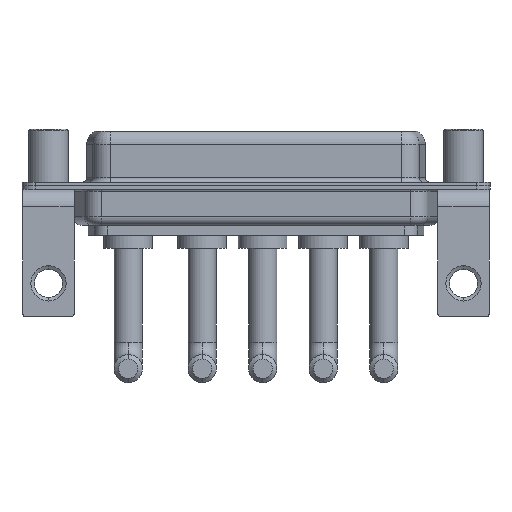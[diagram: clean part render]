
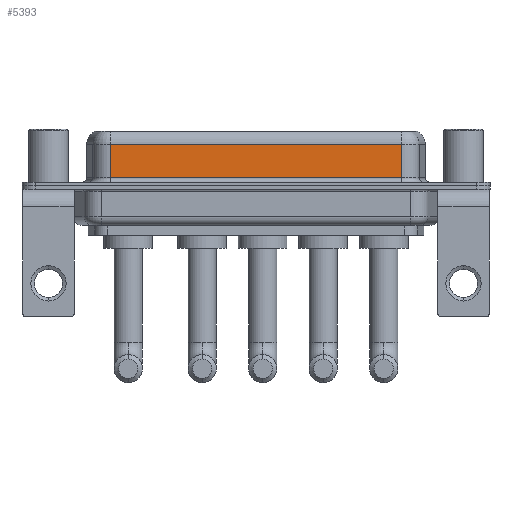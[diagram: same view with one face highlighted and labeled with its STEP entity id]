
A CAD part, front view. The second image highlights one B-rep face of the part: STEP entity #5393.
In plain terms, the highlighted planar face has unit normal (0, -1, 0).
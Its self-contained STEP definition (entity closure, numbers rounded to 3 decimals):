
#1314 = VECTOR ( 'NONE', #11670, 1000. ) ;
#1355 = CARTESIAN_POINT ( 'NONE',  ( 40.037, -3.95, 0.9 ) ) ;
#1744 = PLANE ( 'NONE',  #7026 ) ;
#2052 = CARTESIAN_POINT ( 'NONE',  ( 7.013, -3.95, 0.9 ) ) ;
#2108 = EDGE_CURVE ( 'NONE', #8559, #7716, #10728, .T. ) ;
#2201 = ORIENTED_EDGE ( 'NONE', *, *, #2108, .T. ) ;
#2359 = CARTESIAN_POINT ( 'NONE',  ( 40.037, -3.95, 4.65 ) ) ;
#2680 = VECTOR ( 'NONE', #7348, 1000. ) ;
#4213 = LINE ( 'NONE', #5383, #14626 ) ;
#4260 = EDGE_CURVE ( 'NONE', #7000, #5356, #11518, .T. ) ;
#4943 = EDGE_CURVE ( 'NONE', #8559, #5356, #4213, .T. ) ;
#5019 = CARTESIAN_POINT ( 'NONE',  ( 40.037, -3.95, 4.65 ) ) ;
#5356 = VERTEX_POINT ( 'NONE', #1355 ) ;
#5383 = CARTESIAN_POINT ( 'NONE',  ( 40.037, -3.95, 6.4 ) ) ;
#5393 = ADVANCED_FACE ( 'NONE', ( #11448 ), #1744, .F. ) ;
#5395 = EDGE_LOOP ( 'NONE', ( #12121, #2201, #13074, #6620 ) ) ;
#5891 = VECTOR ( 'NONE', #14658, 1000. ) ;
#6620 = ORIENTED_EDGE ( 'NONE', *, *, #4260, .T. ) ;
#6686 = CARTESIAN_POINT ( 'NONE',  ( 40.037, -3.95, 6.4 ) ) ;
#7000 = VERTEX_POINT ( 'NONE', #2052 ) ;
#7026 = AXIS2_PLACEMENT_3D ( 'NONE', #6686, #9990, #7611 ) ;
#7348 = DIRECTION ( 'NONE',  ( -1., 0., 0. ) ) ;
#7611 = DIRECTION ( 'NONE',  ( 0., 0., 1. ) ) ;
#7716 = VERTEX_POINT ( 'NONE', #15023 ) ;
#8559 = VERTEX_POINT ( 'NONE', #2359 ) ;
#8659 = CARTESIAN_POINT ( 'NONE',  ( 7.013, -3.95, 6.4 ) ) ;
#9150 = EDGE_CURVE ( 'NONE', #7716, #7000, #14499, .T. ) ;
#9220 = CARTESIAN_POINT ( 'NONE',  ( 40.037, -3.95, 0.9 ) ) ;
#9990 = DIRECTION ( 'NONE',  ( 0., 1., 0. ) ) ;
#10728 = LINE ( 'NONE', #5019, #2680 ) ;
#11448 = FACE_OUTER_BOUND ( 'NONE', #5395, .T. ) ;
#11518 = LINE ( 'NONE', #9220, #1314 ) ;
#11670 = DIRECTION ( 'NONE',  ( 1., 0., 0. ) ) ;
#12121 = ORIENTED_EDGE ( 'NONE', *, *, #4943, .F. ) ;
#13074 = ORIENTED_EDGE ( 'NONE', *, *, #9150, .T. ) ;
#13617 = DIRECTION ( 'NONE',  ( 0., 0., -1. ) ) ;
#14499 = LINE ( 'NONE', #8659, #5891 ) ;
#14626 = VECTOR ( 'NONE', #13617, 1000. ) ;
#14658 = DIRECTION ( 'NONE',  ( 0., 0., -1. ) ) ;
#15023 = CARTESIAN_POINT ( 'NONE',  ( 7.013, -3.95, 4.65 ) ) ;
